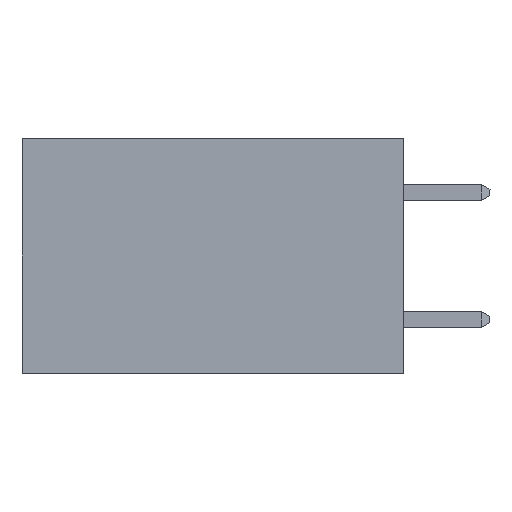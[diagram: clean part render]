
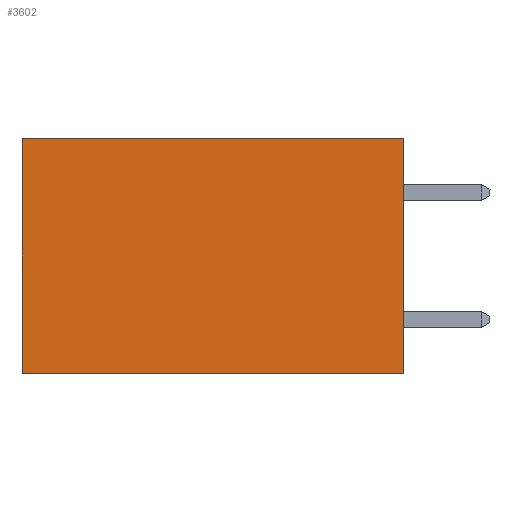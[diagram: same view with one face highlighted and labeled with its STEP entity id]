
A CAD part, left-side view. The second image highlights one B-rep face of the part: STEP entity #3602.
In plain terms, the highlighted planar face has unit normal (-1, 0, 0).
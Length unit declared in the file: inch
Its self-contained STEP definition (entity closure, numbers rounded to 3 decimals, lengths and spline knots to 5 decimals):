
#80 = CARTESIAN_POINT ( 'NONE',  ( 0.2875, 0., 0. ) ) ;
#202 = CARTESIAN_POINT ( 'NONE',  ( 0.2875, 0.6, 0. ) ) ;
#226 = VERTEX_POINT ( 'NONE', #80 ) ;
#495 = EDGE_CURVE ( 'NONE', #10884, #7805, #781, .T. ) ;
#598 = VERTEX_POINT ( 'NONE', #1952 ) ;
#781 = LINE ( 'NONE', #8016, #7631 ) ;
#975 = DIRECTION ( 'NONE',  ( 0., 1., 0. ) ) ;
#1081 = LINE ( 'NONE', #202, #3958 ) ;
#1522 = EDGE_LOOP ( 'NONE', ( #8190, #7506, #8877, #4002 ) ) ;
#1952 = CARTESIAN_POINT ( 'NONE',  ( 0.2875, 0.6, 0. ) ) ;
#1988 = VECTOR ( 'NONE', #5249, 39.37008 ) ;
#2393 = CARTESIAN_POINT ( 'NONE',  ( 0.2875, 0., 0. ) ) ;
#2548 = EDGE_CURVE ( 'NONE', #226, #10884, #10682, .T. ) ;
#3096 = DIRECTION ( 'NONE',  ( 0., 0., -1. ) ) ;
#3602 = ADVANCED_FACE ( 'NONE', ( #4777 ), #9043, .F. ) ;
#3958 = VECTOR ( 'NONE', #8957, 39.37008 ) ;
#4002 = ORIENTED_EDGE ( 'NONE', *, *, #6013, .T. ) ;
#4319 = LINE ( 'NONE', #2393, #1988 ) ;
#4377 = EDGE_CURVE ( 'NONE', #598, #7805, #1081, .T. ) ;
#4777 = FACE_OUTER_BOUND ( 'NONE', #1522, .T. ) ;
#4842 = CARTESIAN_POINT ( 'NONE',  ( 0.2875, 0., 0. ) ) ;
#5249 = DIRECTION ( 'NONE',  ( 0., 1., 0. ) ) ;
#6013 = EDGE_CURVE ( 'NONE', #226, #598, #4319, .T. ) ;
#6468 = AXIS2_PLACEMENT_3D ( 'NONE', #7281, #10807, #7238 ) ;
#7238 = DIRECTION ( 'NONE',  ( 0., 0., -1. ) ) ;
#7281 = CARTESIAN_POINT ( 'NONE',  ( 0.2875, 0., 0. ) ) ;
#7506 = ORIENTED_EDGE ( 'NONE', *, *, #495, .F. ) ;
#7580 = VECTOR ( 'NONE', #3096, 39.37008 ) ;
#7631 = VECTOR ( 'NONE', #975, 39.37008 ) ;
#7805 = VERTEX_POINT ( 'NONE', #8850 ) ;
#8016 = CARTESIAN_POINT ( 'NONE',  ( 0.2875, 0., -0.37 ) ) ;
#8190 = ORIENTED_EDGE ( 'NONE', *, *, #4377, .T. ) ;
#8850 = CARTESIAN_POINT ( 'NONE',  ( 0.2875, 0.6, -0.37 ) ) ;
#8877 = ORIENTED_EDGE ( 'NONE', *, *, #2548, .F. ) ;
#8957 = DIRECTION ( 'NONE',  ( 0., 0., -1. ) ) ;
#9043 = PLANE ( 'NONE',  #6468 ) ;
#9637 = CARTESIAN_POINT ( 'NONE',  ( 0.2875, 0., -0.37 ) ) ;
#10682 = LINE ( 'NONE', #4842, #7580 ) ;
#10807 = DIRECTION ( 'NONE',  ( 1., 0., 0. ) ) ;
#10884 = VERTEX_POINT ( 'NONE', #9637 ) ;
